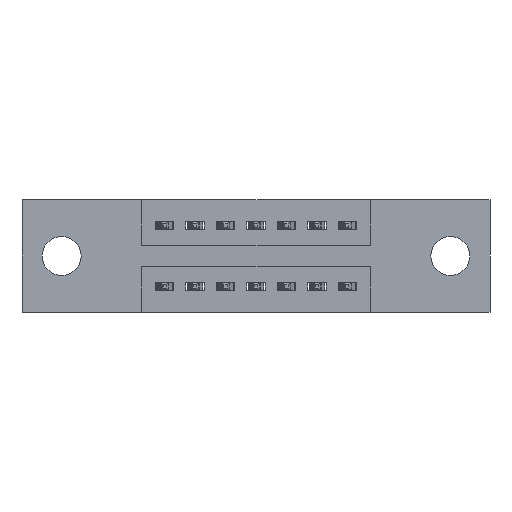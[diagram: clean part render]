
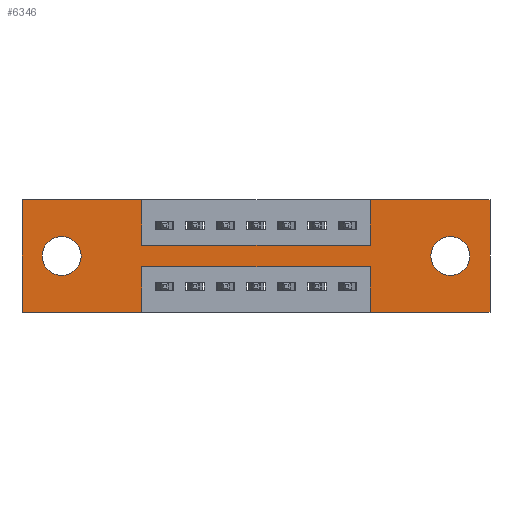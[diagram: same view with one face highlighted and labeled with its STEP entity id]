
A CAD part, front view. The second image highlights one B-rep face of the part: STEP entity #6346.
In plain terms, the highlighted planar face has unit normal (0, -1, 0).
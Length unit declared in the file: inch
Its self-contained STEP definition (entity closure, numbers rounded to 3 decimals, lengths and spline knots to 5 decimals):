
#27 = VECTOR ( 'NONE', #1581, 39.37008 ) ;
#31 = EDGE_LOOP ( 'NONE', ( #2924, #3440 ) ) ;
#63 = ORIENTED_EDGE ( 'NONE', *, *, #9033, .F. ) ;
#318 = CARTESIAN_POINT ( 'NONE',  ( 0.3925, 0., 0. ) ) ;
#326 = VERTEX_POINT ( 'NONE', #610 ) ;
#333 = ORIENTED_EDGE ( 'NONE', *, *, #2013, .F. ) ;
#408 = ORIENTED_EDGE ( 'NONE', *, *, #9071, .F. ) ;
#429 = VECTOR ( 'NONE', #645, 39.37008 ) ;
#431 = ORIENTED_EDGE ( 'NONE', *, *, #4465, .F. ) ;
#473 = ORIENTED_EDGE ( 'NONE', *, *, #6560, .F. ) ;
#565 = LINE ( 'NONE', #7687, #4706 ) ;
#610 = CARTESIAN_POINT ( 'NONE',  ( 1.535, 0., 0. ) ) ;
#645 = DIRECTION ( 'NONE',  ( -1., 0., 0. ) ) ;
#752 = CARTESIAN_POINT ( 'NONE',  ( 0., 0., -0.37 ) ) ;
#759 = DIRECTION ( 'NONE',  ( -1., 0., 0. ) ) ;
#823 = VERTEX_POINT ( 'NONE', #8521 ) ;
#865 = CIRCLE ( 'NONE', #4124, 0.064 ) ;
#934 = AXIS2_PLACEMENT_3D ( 'NONE', #9462, #4862, #10164 ) ;
#936 = LINE ( 'NONE', #9909, #9151 ) ;
#939 = LINE ( 'NONE', #7078, #5074 ) ;
#998 = ORIENTED_EDGE ( 'NONE', *, *, #1914, .F. ) ;
#1099 = ORIENTED_EDGE ( 'NONE', *, *, #9746, .F. ) ;
#1135 = EDGE_LOOP ( 'NONE', ( #1467, #6335, #6591, #9249, #63, #333, #4681, #408, #431, #473, #998, #1099 ) ) ;
#1290 = VERTEX_POINT ( 'NONE', #3515 ) ;
#1467 = ORIENTED_EDGE ( 'NONE', *, *, #9978, .F. ) ;
#1474 = VERTEX_POINT ( 'NONE', #9454 ) ;
#1499 = DIRECTION ( 'NONE',  ( 0., 1., 0. ) ) ;
#1581 = DIRECTION ( 'NONE',  ( 1., 0., 0. ) ) ;
#1790 = VERTEX_POINT ( 'NONE', #8291 ) ;
#1870 = CARTESIAN_POINT ( 'NONE',  ( 1.405, 0., -0.185 ) ) ;
#1914 = EDGE_CURVE ( 'NONE', #9697, #6207, #9517, .T. ) ;
#1977 = AXIS2_PLACEMENT_3D ( 'NONE', #3991, #9403, #4794 ) ;
#2013 = EDGE_CURVE ( 'NONE', #2024, #326, #565, .T. ) ;
#2024 = VERTEX_POINT ( 'NONE', #7661 ) ;
#2178 = EDGE_CURVE ( 'NONE', #3069, #1474, #9397, .T. ) ;
#2336 = DIRECTION ( 'NONE',  ( 0., 0., 1. ) ) ;
#2389 = VERTEX_POINT ( 'NONE', #2988 ) ;
#2425 = CARTESIAN_POINT ( 'NONE',  ( 1.1425, 0., -0.37 ) ) ;
#2631 = LINE ( 'NONE', #752, #8651 ) ;
#2674 = VERTEX_POINT ( 'NONE', #318 ) ;
#2710 = DIRECTION ( 'NONE',  ( 0., 0., -1. ) ) ;
#2794 = VERTEX_POINT ( 'NONE', #5576 ) ;
#2841 = DIRECTION ( 'NONE',  ( 0., 0., -1. ) ) ;
#2924 = ORIENTED_EDGE ( 'NONE', *, *, #9800, .T. ) ;
#2988 = CARTESIAN_POINT ( 'NONE',  ( 1.405, 0., -0.249 ) ) ;
#3003 = AXIS2_PLACEMENT_3D ( 'NONE', #9223, #9937, #5427 ) ;
#3015 = VERTEX_POINT ( 'NONE', #9429 ) ;
#3033 = DIRECTION ( 'NONE',  ( 1., 0., 0. ) ) ;
#3069 = VERTEX_POINT ( 'NONE', #8374 ) ;
#3083 = CIRCLE ( 'NONE', #1977, 0.064 ) ;
#3124 = CARTESIAN_POINT ( 'NONE',  ( 0., 0., -0.37 ) ) ;
#3131 = EDGE_CURVE ( 'NONE', #1290, #2024, #939, .T. ) ;
#3209 = VECTOR ( 'NONE', #5590, 39.37008 ) ;
#3276 = CARTESIAN_POINT ( 'NONE',  ( 0., 0., 0. ) ) ;
#3395 = EDGE_LOOP ( 'NONE', ( #10135, #6707 ) ) ;
#3440 = ORIENTED_EDGE ( 'NONE', *, *, #9739, .T. ) ;
#3482 = EDGE_CURVE ( 'NONE', #8141, #3069, #6202, .T. ) ;
#3515 = CARTESIAN_POINT ( 'NONE',  ( 1.1425, 0., -0.15 ) ) ;
#3568 = CARTESIAN_POINT ( 'NONE',  ( 0.3925, 0., -0.37 ) ) ;
#3783 = PLANE ( 'NONE',  #3003 ) ;
#3790 = DIRECTION ( 'NONE',  ( 0., 0., -1. ) ) ;
#3934 = DIRECTION ( 'NONE',  ( 0., 0., -1. ) ) ;
#3991 = CARTESIAN_POINT ( 'NONE',  ( 1.405, 0., -0.185 ) ) ;
#3999 = CARTESIAN_POINT ( 'NONE',  ( 0.3925, 0., 0. ) ) ;
#4029 = VECTOR ( 'NONE', #2336, 39.37008 ) ;
#4124 = AXIS2_PLACEMENT_3D ( 'NONE', #1870, #7455, #2710 ) ;
#4351 = FACE_BOUND ( 'NONE', #3395, .T. ) ;
#4465 = EDGE_CURVE ( 'NONE', #2674, #1790, #5421, .T. ) ;
#4681 = ORIENTED_EDGE ( 'NONE', *, *, #3131, .F. ) ;
#4706 = VECTOR ( 'NONE', #7631, 39.37008 ) ;
#4749 = EDGE_CURVE ( 'NONE', #823, #8141, #2631, .T. ) ;
#4794 = DIRECTION ( 'NONE',  ( 0., 0., -1. ) ) ;
#4799 = VECTOR ( 'NONE', #3033, 39.37008 ) ;
#4862 = DIRECTION ( 'NONE',  ( 0., 1., 0. ) ) ;
#4956 = CARTESIAN_POINT ( 'NONE',  ( 0.13, 0., -0.121 ) ) ;
#5074 = VECTOR ( 'NONE', #7055, 39.37008 ) ;
#5162 = VECTOR ( 'NONE', #3934, 39.37008 ) ;
#5421 = LINE ( 'NONE', #3999, #5162 ) ;
#5427 = DIRECTION ( 'NONE',  ( 0., 0., -1. ) ) ;
#5483 = VECTOR ( 'NONE', #8270, 39.37008 ) ;
#5506 = VERTEX_POINT ( 'NONE', #3568 ) ;
#5568 = CARTESIAN_POINT ( 'NONE',  ( 0.3925, 0., -0.22 ) ) ;
#5576 = CARTESIAN_POINT ( 'NONE',  ( 0.13, 0., -0.249 ) ) ;
#5590 = DIRECTION ( 'NONE',  ( -1., 0., 0. ) ) ;
#6024 = VERTEX_POINT ( 'NONE', #4956 ) ;
#6056 = CARTESIAN_POINT ( 'NONE',  ( 0.3925, 0., -0.37 ) ) ;
#6111 = EDGE_CURVE ( 'NONE', #2389, #3015, #865, .T. ) ;
#6202 = LINE ( 'NONE', #2425, #4029 ) ;
#6207 = VERTEX_POINT ( 'NONE', #7549 ) ;
#6335 = ORIENTED_EDGE ( 'NONE', *, *, #2178, .F. ) ;
#6346 = ADVANCED_FACE ( 'NONE', ( #4351, #8503, #6507 ), #3783, .T. ) ;
#6398 = CARTESIAN_POINT ( 'NONE',  ( 0.13, 0., -0.185 ) ) ;
#6507 = FACE_OUTER_BOUND ( 'NONE', #1135, .T. ) ;
#6560 = EDGE_CURVE ( 'NONE', #6207, #2674, #6631, .T. ) ;
#6591 = ORIENTED_EDGE ( 'NONE', *, *, #3482, .F. ) ;
#6631 = LINE ( 'NONE', #3276, #27 ) ;
#6707 = ORIENTED_EDGE ( 'NONE', *, *, #6111, .T. ) ;
#6944 = LINE ( 'NONE', #9264, #4799 ) ;
#7055 = DIRECTION ( 'NONE',  ( 0., 0., 1. ) ) ;
#7078 = CARTESIAN_POINT ( 'NONE',  ( 1.1425, 0., 0. ) ) ;
#7165 = DIRECTION ( 'NONE',  ( 0., 0., 1. ) ) ;
#7183 = CIRCLE ( 'NONE', #8642, 0.064 ) ;
#7415 = CARTESIAN_POINT ( 'NONE',  ( 1.1425, 0., -0.37 ) ) ;
#7455 = DIRECTION ( 'NONE',  ( 0., 1., 0. ) ) ;
#7549 = CARTESIAN_POINT ( 'NONE',  ( 0., 0., 0. ) ) ;
#7631 = DIRECTION ( 'NONE',  ( 1., 0., 0. ) ) ;
#7661 = CARTESIAN_POINT ( 'NONE',  ( 1.1425, 0., 0. ) ) ;
#7687 = CARTESIAN_POINT ( 'NONE',  ( 0., 0., 0. ) ) ;
#7925 = EDGE_CURVE ( 'NONE', #3015, #2389, #3083, .T. ) ;
#8141 = VERTEX_POINT ( 'NONE', #7415 ) ;
#8222 = CIRCLE ( 'NONE', #934, 0.064 ) ;
#8270 = DIRECTION ( 'NONE',  ( 0., 0., 1. ) ) ;
#8291 = CARTESIAN_POINT ( 'NONE',  ( 0.3925, 0., -0.15 ) ) ;
#8337 = VECTOR ( 'NONE', #2841, 39.37008 ) ;
#8374 = CARTESIAN_POINT ( 'NONE',  ( 1.1425, 0., -0.22 ) ) ;
#8413 = CARTESIAN_POINT ( 'NONE',  ( 0., 0., 0. ) ) ;
#8503 = FACE_BOUND ( 'NONE', #31, .T. ) ;
#8521 = CARTESIAN_POINT ( 'NONE',  ( 1.535, 0., -0.37 ) ) ;
#8588 = LINE ( 'NONE', #6056, #8337 ) ;
#8642 = AXIS2_PLACEMENT_3D ( 'NONE', #6398, #1499, #7165 ) ;
#8651 = VECTOR ( 'NONE', #759, 39.37008 ) ;
#8937 = LINE ( 'NONE', #10075, #429 ) ;
#9033 = EDGE_CURVE ( 'NONE', #326, #823, #936, .T. ) ;
#9071 = EDGE_CURVE ( 'NONE', #1790, #1290, #6944, .T. ) ;
#9151 = VECTOR ( 'NONE', #3790, 39.37008 ) ;
#9223 = CARTESIAN_POINT ( 'NONE',  ( 0., 0., -0.37 ) ) ;
#9249 = ORIENTED_EDGE ( 'NONE', *, *, #4749, .F. ) ;
#9264 = CARTESIAN_POINT ( 'NONE',  ( 0.3925, 0., -0.15 ) ) ;
#9397 = LINE ( 'NONE', #5568, #3209 ) ;
#9403 = DIRECTION ( 'NONE',  ( 0., 1., 0. ) ) ;
#9429 = CARTESIAN_POINT ( 'NONE',  ( 1.405, 0., -0.121 ) ) ;
#9454 = CARTESIAN_POINT ( 'NONE',  ( 0.3925, 0., -0.22 ) ) ;
#9462 = CARTESIAN_POINT ( 'NONE',  ( 0.13, 0., -0.185 ) ) ;
#9517 = LINE ( 'NONE', #8413, #5483 ) ;
#9697 = VERTEX_POINT ( 'NONE', #3124 ) ;
#9739 = EDGE_CURVE ( 'NONE', #2794, #6024, #7183, .T. ) ;
#9746 = EDGE_CURVE ( 'NONE', #5506, #9697, #8937, .T. ) ;
#9800 = EDGE_CURVE ( 'NONE', #6024, #2794, #8222, .T. ) ;
#9909 = CARTESIAN_POINT ( 'NONE',  ( 1.535, 0., 0. ) ) ;
#9937 = DIRECTION ( 'NONE',  ( 0., -1., 0. ) ) ;
#9978 = EDGE_CURVE ( 'NONE', #1474, #5506, #8588, .T. ) ;
#10075 = CARTESIAN_POINT ( 'NONE',  ( 0., 0., -0.37 ) ) ;
#10135 = ORIENTED_EDGE ( 'NONE', *, *, #7925, .T. ) ;
#10164 = DIRECTION ( 'NONE',  ( 0., 0., 1. ) ) ;
